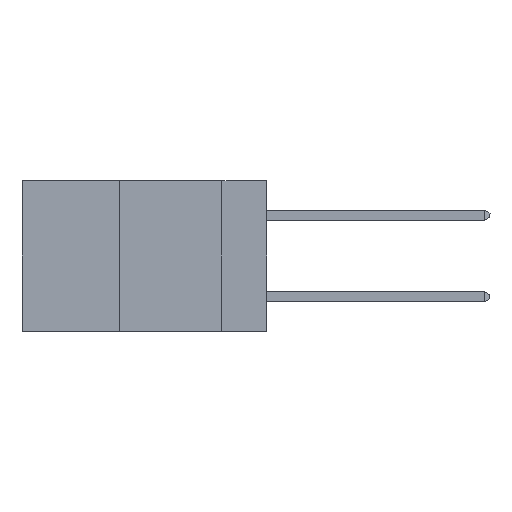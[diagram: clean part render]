
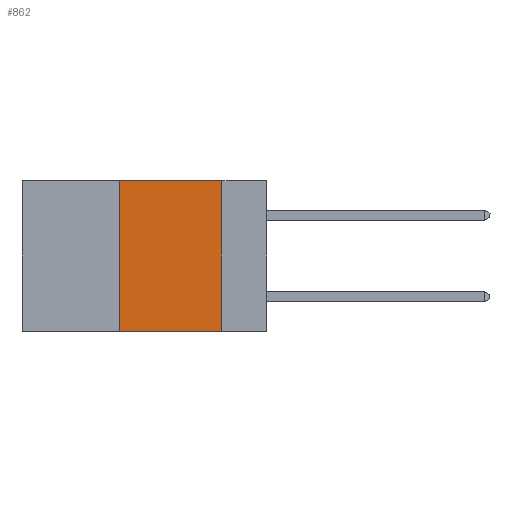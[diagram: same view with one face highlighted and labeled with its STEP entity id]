
A CAD part, left-side view. The second image highlights one B-rep face of the part: STEP entity #862.
In plain terms, the highlighted planar face has unit normal (-1, 0, 0).
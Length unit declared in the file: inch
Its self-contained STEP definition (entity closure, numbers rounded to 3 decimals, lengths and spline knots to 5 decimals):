
#137 = DIRECTION ( 'NONE',  ( 0., -1., 0. ) ) ;
#701 = CARTESIAN_POINT ( 'NONE',  ( 0., 0.11, 0. ) ) ;
#862 = ADVANCED_FACE ( 'NONE', ( #7032 ), #8339, .F. ) ;
#877 = ORIENTED_EDGE ( 'NONE', *, *, #7917, .F. ) ;
#1671 = ORIENTED_EDGE ( 'NONE', *, *, #6243, .T. ) ;
#1891 = VERTEX_POINT ( 'NONE', #2845 ) ;
#1902 = DIRECTION ( 'NONE',  ( 0., 0., -1. ) ) ;
#2006 = CARTESIAN_POINT ( 'NONE',  ( 0., 0.36, 0. ) ) ;
#2325 = AXIS2_PLACEMENT_3D ( 'NONE', #8436, #8229, #8213 ) ;
#2845 = CARTESIAN_POINT ( 'NONE',  ( 0., 0.11, -0.37 ) ) ;
#3242 = VECTOR ( 'NONE', #1902, 39.37008 ) ;
#4689 = DIRECTION ( 'NONE',  ( 0., -1., 0. ) ) ;
#4733 = VECTOR ( 'NONE', #137, 39.37008 ) ;
#6243 = EDGE_CURVE ( 'NONE', #9323, #1891, #12385, .T. ) ;
#6754 = ORIENTED_EDGE ( 'NONE', *, *, #7863, .F. ) ;
#7032 = FACE_OUTER_BOUND ( 'NONE', #9395, .T. ) ;
#7586 = EDGE_CURVE ( 'NONE', #12348, #1891, #11007, .T. ) ;
#7863 = EDGE_CURVE ( 'NONE', #9323, #8488, #9539, .T. ) ;
#7917 = EDGE_CURVE ( 'NONE', #8488, #12348, #10996, .T. ) ;
#8125 = ORIENTED_EDGE ( 'NONE', *, *, #7586, .F. ) ;
#8213 = DIRECTION ( 'NONE',  ( 0., 0., -1. ) ) ;
#8229 = DIRECTION ( 'NONE',  ( 1., 0., 0. ) ) ;
#8339 = PLANE ( 'NONE',  #2325 ) ;
#8436 = CARTESIAN_POINT ( 'NONE',  ( 0., 0.6, 0. ) ) ;
#8488 = VERTEX_POINT ( 'NONE', #2006 ) ;
#9258 = VECTOR ( 'NONE', #10411, 39.37008 ) ;
#9323 = VERTEX_POINT ( 'NONE', #10554 ) ;
#9395 = EDGE_LOOP ( 'NONE', ( #8125, #877, #6754, #1671 ) ) ;
#9539 = LINE ( 'NONE', #12233, #9258 ) ;
#10411 = DIRECTION ( 'NONE',  ( 0., 0., 1. ) ) ;
#10517 = CARTESIAN_POINT ( 'NONE',  ( 0., 0.6, 0. ) ) ;
#10554 = CARTESIAN_POINT ( 'NONE',  ( 0., 0.36, -0.37 ) ) ;
#10730 = VECTOR ( 'NONE', #4689, 39.37008 ) ;
#10996 = LINE ( 'NONE', #10517, #10730 ) ;
#11007 = LINE ( 'NONE', #12676, #3242 ) ;
#11072 = CARTESIAN_POINT ( 'NONE',  ( 0., 0.6, -0.37 ) ) ;
#12233 = CARTESIAN_POINT ( 'NONE',  ( 0., 0.36, 0. ) ) ;
#12348 = VERTEX_POINT ( 'NONE', #701 ) ;
#12385 = LINE ( 'NONE', #11072, #4733 ) ;
#12676 = CARTESIAN_POINT ( 'NONE',  ( 0., 0.11, 0. ) ) ;
